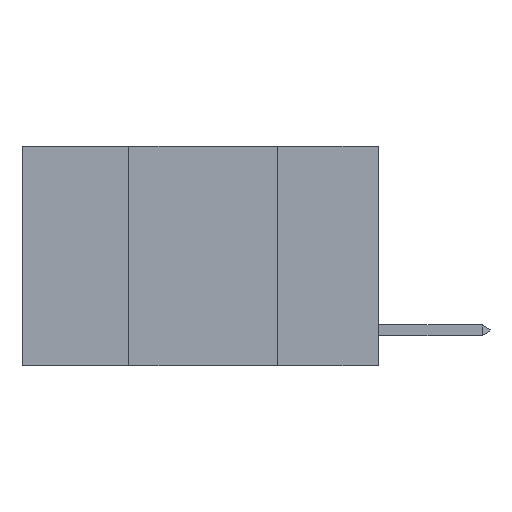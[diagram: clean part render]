
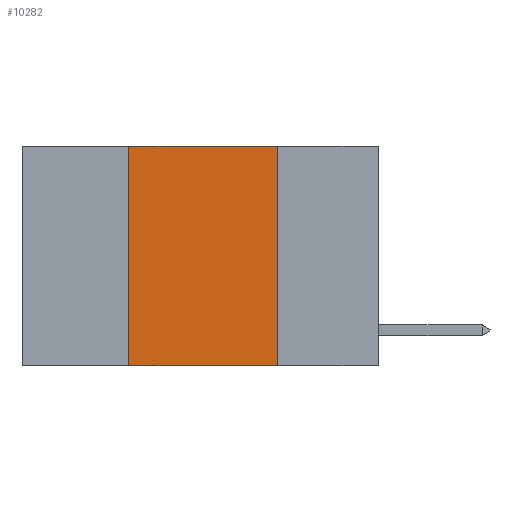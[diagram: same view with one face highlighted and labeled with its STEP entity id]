
A CAD part, left-side view. The second image highlights one B-rep face of the part: STEP entity #10282.
In plain terms, the highlighted planar face has unit normal (-1, 0, 0).
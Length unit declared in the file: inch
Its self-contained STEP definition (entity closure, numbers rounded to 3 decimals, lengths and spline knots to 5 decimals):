
#104 = CARTESIAN_POINT ( 'NONE',  ( 0., 0.6, 0. ) ) ;
#264 = LINE ( 'NONE', #6459, #2354 ) ;
#690 = DIRECTION ( 'NONE',  ( 0., 0., 1. ) ) ;
#804 = CARTESIAN_POINT ( 'NONE',  ( 0., 0.6, -0.37 ) ) ;
#2032 = CARTESIAN_POINT ( 'NONE',  ( 0., 0.42, 0. ) ) ;
#2354 = VECTOR ( 'NONE', #11142, 39.37008 ) ;
#3170 = CARTESIAN_POINT ( 'NONE',  ( 0., 0.42, 0. ) ) ;
#4013 = VERTEX_POINT ( 'NONE', #9214 ) ;
#4285 = EDGE_CURVE ( 'NONE', #4931, #14768, #264, .T. ) ;
#4491 = EDGE_CURVE ( 'NONE', #4013, #14768, #14951, .T. ) ;
#4835 = VECTOR ( 'NONE', #9120, 39.37008 ) ;
#4931 = VERTEX_POINT ( 'NONE', #11826 ) ;
#5097 = CARTESIAN_POINT ( 'NONE',  ( 0., 0.6, 0. ) ) ;
#5251 = VECTOR ( 'NONE', #690, 39.37008 ) ;
#5346 = EDGE_LOOP ( 'NONE', ( #13981, #13136, #14536, #5351 ) ) ;
#5351 = ORIENTED_EDGE ( 'NONE', *, *, #4491, .T. ) ;
#6351 = VECTOR ( 'NONE', #11998, 39.37008 ) ;
#6449 = VERTEX_POINT ( 'NONE', #2032 ) ;
#6459 = CARTESIAN_POINT ( 'NONE',  ( 0., 0.17, 0. ) ) ;
#9120 = DIRECTION ( 'NONE',  ( 0., -1., 0. ) ) ;
#9214 = CARTESIAN_POINT ( 'NONE',  ( 0., 0.42, -0.37 ) ) ;
#10282 = ADVANCED_FACE ( 'NONE', ( #12896 ), #14142, .F. ) ;
#10456 = EDGE_CURVE ( 'NONE', #4013, #6449, #11323, .T. ) ;
#10618 = LINE ( 'NONE', #104, #6351 ) ;
#10947 = DIRECTION ( 'NONE',  ( 0., 0., -1. ) ) ;
#10984 = AXIS2_PLACEMENT_3D ( 'NONE', #5097, #12258, #10947 ) ;
#11142 = DIRECTION ( 'NONE',  ( 0., 0., -1. ) ) ;
#11323 = LINE ( 'NONE', #3170, #5251 ) ;
#11697 = CARTESIAN_POINT ( 'NONE',  ( 0., 0.17, -0.37 ) ) ;
#11826 = CARTESIAN_POINT ( 'NONE',  ( 0., 0.17, 0. ) ) ;
#11998 = DIRECTION ( 'NONE',  ( 0., -1., 0. ) ) ;
#12258 = DIRECTION ( 'NONE',  ( 1., 0., 0. ) ) ;
#12896 = FACE_OUTER_BOUND ( 'NONE', #5346, .T. ) ;
#13136 = ORIENTED_EDGE ( 'NONE', *, *, #14954, .F. ) ;
#13981 = ORIENTED_EDGE ( 'NONE', *, *, #4285, .F. ) ;
#14142 = PLANE ( 'NONE',  #10984 ) ;
#14536 = ORIENTED_EDGE ( 'NONE', *, *, #10456, .F. ) ;
#14768 = VERTEX_POINT ( 'NONE', #11697 ) ;
#14951 = LINE ( 'NONE', #804, #4835 ) ;
#14954 = EDGE_CURVE ( 'NONE', #6449, #4931, #10618, .T. ) ;
